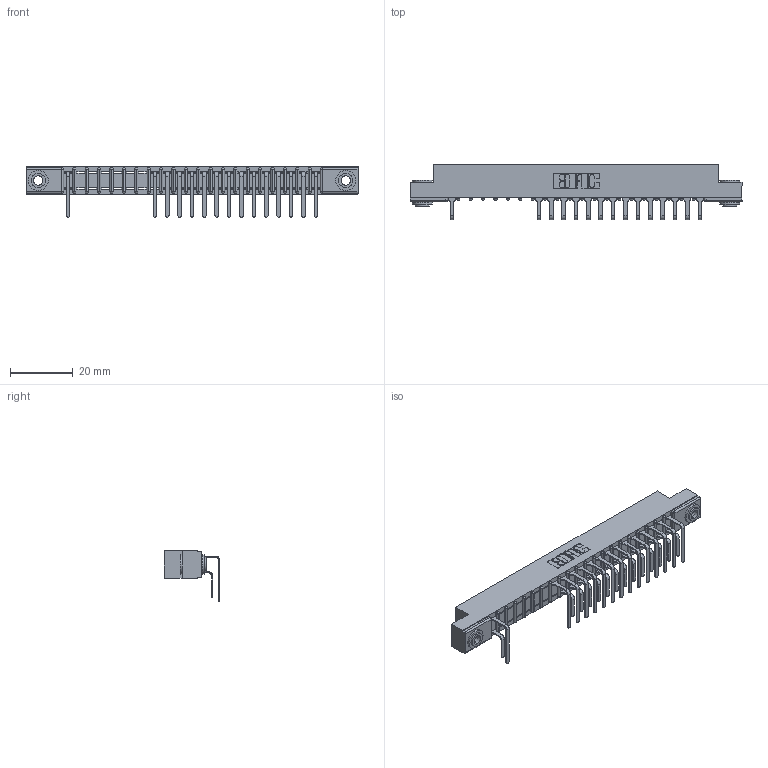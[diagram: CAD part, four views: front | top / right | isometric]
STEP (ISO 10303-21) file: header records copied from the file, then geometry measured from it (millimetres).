
FILE_DESCRIPTION (( 'STEP AP203' ), '1' );
FILE_NAME ('307-042-559-203.STEP', '2018-08-05T18:38:54', ( '' ), ( '' ), 'SwSTEP 2.0', 'SolidWorks 2016', '' );
FILE_SCHEMA (( 'CONFIG_CONTROL_DESIGN' ));
Length unit declared in the file: inch
Products named in the file (5): 307 Part_.156 Dia Mounting Holes; 307-290-001_558 559 - 1 (Single); 307-290-001_559 - 2 (Single); 345-250-002_345-250-002-102; 307-042-559-203
Assembly tree (32 placements, depth 2):
  307-042-559-203
    307 Part_.156 Dia Mounting Holes
    307-290-001_558 559 - 1 (Single)  x14
    307-290-001_559 - 2 (Single)  x15
    345-250-002_345-250-002-102  x2
Bounding box: 106.22 x 17.69 x 16.08 mm (x, y, z)
Volume: 6911.4 mm3; surface area: 12142.1 mm2
Topology: 32 solids, 32 shells, 1772 faces, 4969 edges, 3210 vertices
Faces by surface type: plane 1129, cylinder 591, sphere 44, cone 8
Entity records: 23360 total; most frequent: CARTESIAN_POINT 3867, ORIENTED_EDGE 3834, DIRECTION 3797, EDGE_CURVE 1917, LINE 1453, VECTOR 1453, VERTEX_POINT 1242, AXIS2_PLACEMENT_3D 1172
